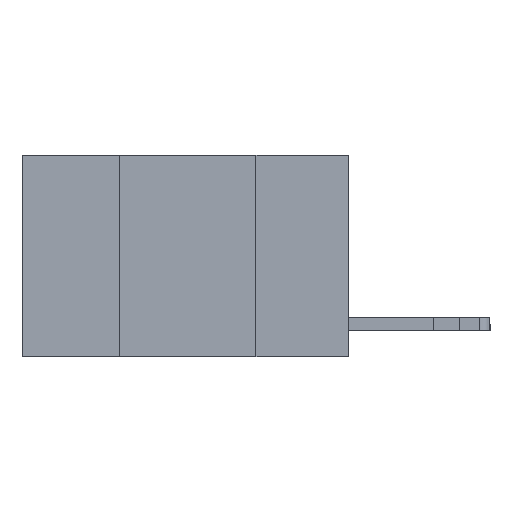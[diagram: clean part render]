
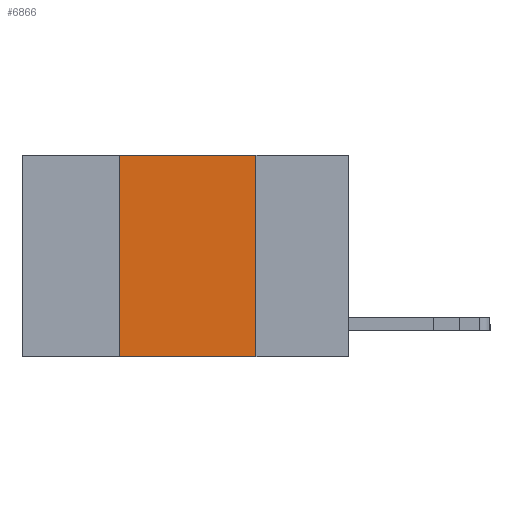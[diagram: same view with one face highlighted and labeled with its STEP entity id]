
A CAD part, left-side view. The second image highlights one B-rep face of the part: STEP entity #6866.
In plain terms, the highlighted planar face has unit normal (-1, 0, 0).
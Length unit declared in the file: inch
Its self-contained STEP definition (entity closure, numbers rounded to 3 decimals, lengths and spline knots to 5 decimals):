
#129 = DIRECTION ( 'NONE',  ( 0., -1., 0. ) ) ;
#164 = CARTESIAN_POINT ( 'NONE',  ( 0., 0.42, 0. ) ) ;
#355 = VECTOR ( 'NONE', #3787, 39.37008 ) ;
#432 = CARTESIAN_POINT ( 'NONE',  ( 0., 0.6, 0. ) ) ;
#1171 = LINE ( 'NONE', #5788, #6151 ) ;
#1777 = DIRECTION ( 'NONE',  ( 0., 0., -1. ) ) ;
#2317 = ORIENTED_EDGE ( 'NONE', *, *, #3573, .T. ) ;
#3359 = LINE ( 'NONE', #5800, #14868 ) ;
#3573 = EDGE_CURVE ( 'NONE', #8833, #7331, #3761, .T. ) ;
#3761 = LINE ( 'NONE', #4903, #4892 ) ;
#3787 = DIRECTION ( 'NONE',  ( 0., 0., 1. ) ) ;
#4727 = AXIS2_PLACEMENT_3D ( 'NONE', #432, #13222, #1777 ) ;
#4827 = ORIENTED_EDGE ( 'NONE', *, *, #8354, .F. ) ;
#4892 = VECTOR ( 'NONE', #5887, 39.37008 ) ;
#4903 = CARTESIAN_POINT ( 'NONE',  ( 0., 0.6, -0.37 ) ) ;
#4927 = LINE ( 'NONE', #164, #355 ) ;
#5597 = VERTEX_POINT ( 'NONE', #6325 ) ;
#5788 = CARTESIAN_POINT ( 'NONE',  ( 0., 0.17, 0. ) ) ;
#5800 = CARTESIAN_POINT ( 'NONE',  ( 0., 0.6, 0. ) ) ;
#5887 = DIRECTION ( 'NONE',  ( 0., -1., 0. ) ) ;
#6151 = VECTOR ( 'NONE', #9259, 39.37008 ) ;
#6186 = PLANE ( 'NONE',  #4727 ) ;
#6325 = CARTESIAN_POINT ( 'NONE',  ( 0., 0.17, 0. ) ) ;
#6866 = ADVANCED_FACE ( 'NONE', ( #14276 ), #6186, .F. ) ;
#7189 = ORIENTED_EDGE ( 'NONE', *, *, #13529, .F. ) ;
#7331 = VERTEX_POINT ( 'NONE', #12691 ) ;
#8177 = VERTEX_POINT ( 'NONE', #9090 ) ;
#8354 = EDGE_CURVE ( 'NONE', #8833, #8177, #4927, .T. ) ;
#8441 = ORIENTED_EDGE ( 'NONE', *, *, #8669, .F. ) ;
#8669 = EDGE_CURVE ( 'NONE', #8177, #5597, #3359, .T. ) ;
#8833 = VERTEX_POINT ( 'NONE', #10099 ) ;
#9090 = CARTESIAN_POINT ( 'NONE',  ( 0., 0.42, 0. ) ) ;
#9259 = DIRECTION ( 'NONE',  ( 0., 0., -1. ) ) ;
#10099 = CARTESIAN_POINT ( 'NONE',  ( 0., 0.42, -0.37 ) ) ;
#12691 = CARTESIAN_POINT ( 'NONE',  ( 0., 0.17, -0.37 ) ) ;
#12911 = EDGE_LOOP ( 'NONE', ( #7189, #8441, #4827, #2317 ) ) ;
#13222 = DIRECTION ( 'NONE',  ( 1., 0., 0. ) ) ;
#13529 = EDGE_CURVE ( 'NONE', #5597, #7331, #1171, .T. ) ;
#14276 = FACE_OUTER_BOUND ( 'NONE', #12911, .T. ) ;
#14868 = VECTOR ( 'NONE', #129, 39.37008 ) ;
